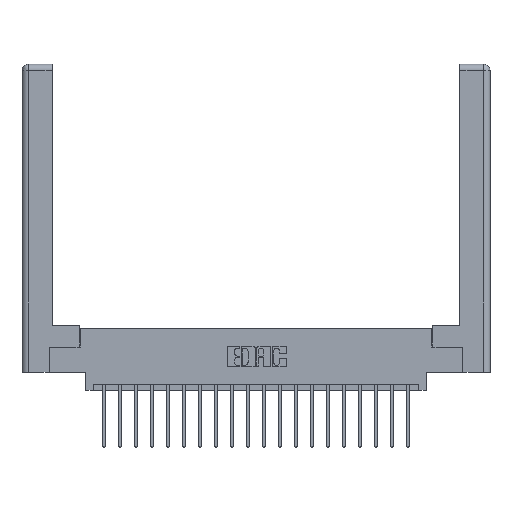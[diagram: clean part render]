
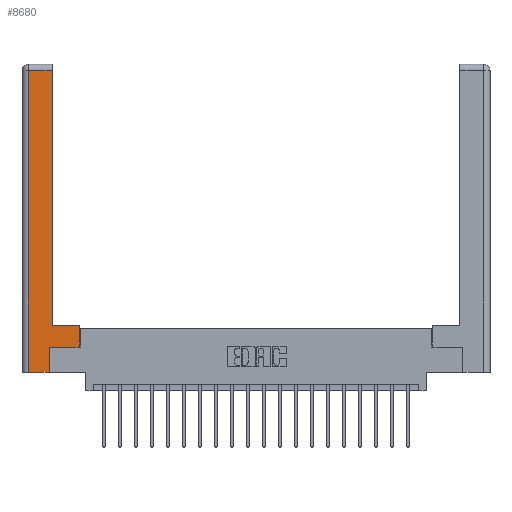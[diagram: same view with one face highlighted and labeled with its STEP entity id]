
A CAD part, top view. The second image highlights one B-rep face of the part: STEP entity #8680.
In plain terms, the highlighted planar face has unit normal (0, 0, 1).
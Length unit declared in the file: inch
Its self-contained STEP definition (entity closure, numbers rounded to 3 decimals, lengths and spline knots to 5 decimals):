
#489 = ORIENTED_EDGE ( 'NONE', *, *, #819, .T. ) ;
#577 = ORIENTED_EDGE ( 'NONE', *, *, #2712, .T. ) ;
#734 = CARTESIAN_POINT ( 'NONE',  ( 0.0615, 0., 0. ) ) ;
#819 = EDGE_CURVE ( 'NONE', #20404, #14229, #4690, .T. ) ;
#1039 = LINE ( 'NONE', #9313, #19724 ) ;
#1040 = DIRECTION ( 'NONE',  ( -1., 0., 0. ) ) ;
#1057 = FACE_OUTER_BOUND ( 'NONE', #20304, .T. ) ;
#1167 = DIRECTION ( 'NONE',  ( -1., 0., 0. ) ) ;
#1333 = VERTEX_POINT ( 'NONE', #3223 ) ;
#2129 = CARTESIAN_POINT ( 'NONE',  ( 0.565, 0.245, 0. ) ) ;
#2166 = VERTEX_POINT ( 'NONE', #8901 ) ;
#2712 = EDGE_CURVE ( 'NONE', #2166, #20404, #11499, .T. ) ;
#2746 = EDGE_CURVE ( 'NONE', #10584, #9302, #5370, .T. ) ;
#2846 = DIRECTION ( 'NONE',  ( -1., 0., 0. ) ) ;
#2876 = VERTEX_POINT ( 'NONE', #2945 ) ;
#2939 = ORIENTED_EDGE ( 'NONE', *, *, #12503, .T. ) ;
#2945 = CARTESIAN_POINT ( 'NONE',  ( 0.0615, 2.94, 0. ) ) ;
#3195 = DIRECTION ( 'NONE',  ( 0., 1., 0. ) ) ;
#3223 = CARTESIAN_POINT ( 'NONE',  ( 0.0615, 0., 0. ) ) ;
#3428 = ORIENTED_EDGE ( 'NONE', *, *, #11660, .T. ) ;
#3716 = VECTOR ( 'NONE', #17005, 39.37008 ) ;
#3911 = DIRECTION ( 'NONE',  ( 0., 1., 0. ) ) ;
#4264 = EDGE_CURVE ( 'NONE', #9302, #17271, #13953, .T. ) ;
#4309 = CARTESIAN_POINT ( 'NONE',  ( 0.295, 0.45, 0. ) ) ;
#4605 = AXIS2_PLACEMENT_3D ( 'NONE', #4618, #11320, #2846 ) ;
#4618 = CARTESIAN_POINT ( 'NONE',  ( 0., 0., 0. ) ) ;
#4690 = LINE ( 'NONE', #21152, #5208 ) ;
#4767 = CARTESIAN_POINT ( 'NONE',  ( 0.565, 0.45, 0. ) ) ;
#5208 = VECTOR ( 'NONE', #10003, 39.37008 ) ;
#5289 = LINE ( 'NONE', #734, #7826 ) ;
#5370 = LINE ( 'NONE', #4309, #10961 ) ;
#5786 = VECTOR ( 'NONE', #3195, 39.37008 ) ;
#6226 = CARTESIAN_POINT ( 'NONE',  ( 0.265, 0.245, 0. ) ) ;
#6295 = LINE ( 'NONE', #4767, #5786 ) ;
#6694 = EDGE_CURVE ( 'NONE', #1333, #2166, #10583, .T. ) ;
#7822 = CARTESIAN_POINT ( 'NONE',  ( 0.295, 3., 0. ) ) ;
#7826 = VECTOR ( 'NONE', #13981, 39.37008 ) ;
#8680 = ADVANCED_FACE ( 'NONE', ( #1057 ), #11111, .F. ) ;
#8901 = CARTESIAN_POINT ( 'NONE',  ( 0.265, 0., 0. ) ) ;
#9302 = VERTEX_POINT ( 'NONE', #12626 ) ;
#9313 = CARTESIAN_POINT ( 'NONE',  ( 0.0615, 2.94, 0. ) ) ;
#10003 = DIRECTION ( 'NONE',  ( 1., 0., 0. ) ) ;
#10549 = ORIENTED_EDGE ( 'NONE', *, *, #6694, .T. ) ;
#10583 = LINE ( 'NONE', #18653, #3716 ) ;
#10584 = VERTEX_POINT ( 'NONE', #11505 ) ;
#10961 = VECTOR ( 'NONE', #1167, 39.37008 ) ;
#11111 = PLANE ( 'NONE',  #4605 ) ;
#11157 = VECTOR ( 'NONE', #17822, 39.37008 ) ;
#11320 = DIRECTION ( 'NONE',  ( 0., 0., -1. ) ) ;
#11471 = EDGE_CURVE ( 'NONE', #2876, #1333, #5289, .T. ) ;
#11499 = LINE ( 'NONE', #18739, #19168 ) ;
#11505 = CARTESIAN_POINT ( 'NONE',  ( 0.565, 0.45, 0. ) ) ;
#11660 = EDGE_CURVE ( 'NONE', #14229, #10584, #6295, .T. ) ;
#12503 = EDGE_CURVE ( 'NONE', #17271, #2876, #1039, .T. ) ;
#12626 = CARTESIAN_POINT ( 'NONE',  ( 0.295, 0.45, 0. ) ) ;
#13229 = ORIENTED_EDGE ( 'NONE', *, *, #2746, .T. ) ;
#13953 = LINE ( 'NONE', #7822, #11157 ) ;
#13981 = DIRECTION ( 'NONE',  ( 0., -1., 0. ) ) ;
#14229 = VERTEX_POINT ( 'NONE', #2129 ) ;
#14769 = ORIENTED_EDGE ( 'NONE', *, *, #11471, .T. ) ;
#17005 = DIRECTION ( 'NONE',  ( 1., 0., 0. ) ) ;
#17186 = CARTESIAN_POINT ( 'NONE',  ( 0.295, 2.94, 0. ) ) ;
#17271 = VERTEX_POINT ( 'NONE', #17186 ) ;
#17822 = DIRECTION ( 'NONE',  ( 0., 1., 0. ) ) ;
#18272 = ORIENTED_EDGE ( 'NONE', *, *, #4264, .T. ) ;
#18653 = CARTESIAN_POINT ( 'NONE',  ( 0.265, 0., 0. ) ) ;
#18739 = CARTESIAN_POINT ( 'NONE',  ( 0.265, 0.245, 0. ) ) ;
#19168 = VECTOR ( 'NONE', #3911, 39.37008 ) ;
#19724 = VECTOR ( 'NONE', #1040, 39.37008 ) ;
#20304 = EDGE_LOOP ( 'NONE', ( #18272, #2939, #14769, #10549, #577, #489, #3428, #13229 ) ) ;
#20404 = VERTEX_POINT ( 'NONE', #6226 ) ;
#21152 = CARTESIAN_POINT ( 'NONE',  ( 0.565, 0.245, 0. ) ) ;
